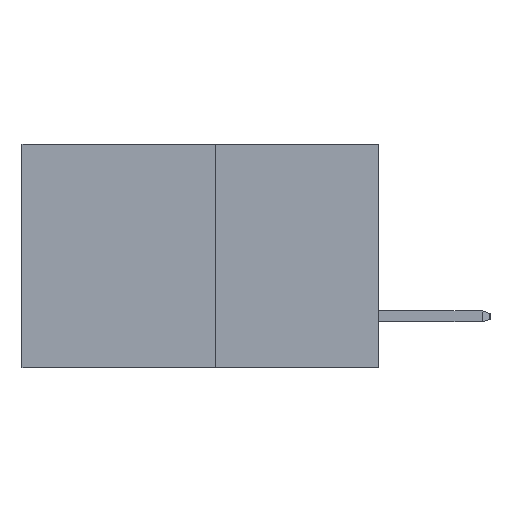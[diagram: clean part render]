
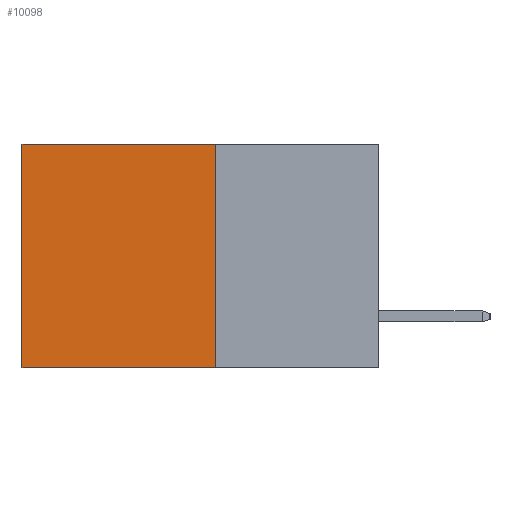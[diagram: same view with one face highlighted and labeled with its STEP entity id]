
A CAD part, left-side view. The second image highlights one B-rep face of the part: STEP entity #10098.
In plain terms, the highlighted planar face has unit normal (-1, 0, 0).
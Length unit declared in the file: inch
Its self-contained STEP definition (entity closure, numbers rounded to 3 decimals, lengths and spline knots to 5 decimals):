
#211 = CARTESIAN_POINT ( 'NONE',  ( 0.277, 0.27, -0.37 ) ) ;
#232 = VERTEX_POINT ( 'NONE', #278 ) ;
#278 = CARTESIAN_POINT ( 'NONE',  ( 0.277, 0.27, 0. ) ) ;
#397 = VECTOR ( 'NONE', #10402, 39.37008 ) ;
#844 = VERTEX_POINT ( 'NONE', #7698 ) ;
#1536 = VERTEX_POINT ( 'NONE', #6334 ) ;
#2068 = CARTESIAN_POINT ( 'NONE',  ( 0.277, 0.27, -0.37 ) ) ;
#2429 = EDGE_CURVE ( 'NONE', #232, #1536, #5053, .T. ) ;
#3121 = CARTESIAN_POINT ( 'NONE',  ( 0.277, 0.59, -0.37 ) ) ;
#3392 = ORIENTED_EDGE ( 'NONE', *, *, #4821, .T. ) ;
#3768 = VECTOR ( 'NONE', #6677, 39.37008 ) ;
#4328 = DIRECTION ( 'NONE',  ( 1., 0., 0. ) ) ;
#4422 = FACE_OUTER_BOUND ( 'NONE', #8122, .T. ) ;
#4745 = EDGE_CURVE ( 'NONE', #232, #7334, #8312, .T. ) ;
#4821 = EDGE_CURVE ( 'NONE', #1536, #844, #9881, .T. ) ;
#5053 = LINE ( 'NONE', #8306, #7510 ) ;
#5304 = ORIENTED_EDGE ( 'NONE', *, *, #4745, .F. ) ;
#5486 = DIRECTION ( 'NONE',  ( 0., 1., 0. ) ) ;
#6055 = AXIS2_PLACEMENT_3D ( 'NONE', #9775, #4328, #10689 ) ;
#6334 = CARTESIAN_POINT ( 'NONE',  ( 0.277, 0.59, 0. ) ) ;
#6677 = DIRECTION ( 'NONE',  ( 0., 0., -1. ) ) ;
#7334 = VERTEX_POINT ( 'NONE', #2068 ) ;
#7510 = VECTOR ( 'NONE', #11266, 39.37008 ) ;
#7698 = CARTESIAN_POINT ( 'NONE',  ( 0.277, 0.59, -0.37 ) ) ;
#7940 = PLANE ( 'NONE',  #6055 ) ;
#8122 = EDGE_LOOP ( 'NONE', ( #3392, #11118, #5304, #11202 ) ) ;
#8306 = CARTESIAN_POINT ( 'NONE',  ( 0.277, 0.27, 0. ) ) ;
#8312 = LINE ( 'NONE', #211, #3768 ) ;
#8406 = EDGE_CURVE ( 'NONE', #7334, #844, #9588, .T. ) ;
#9105 = CARTESIAN_POINT ( 'NONE',  ( 0.277, 0.27, -0.37 ) ) ;
#9304 = VECTOR ( 'NONE', #5486, 39.37008 ) ;
#9588 = LINE ( 'NONE', #9105, #9304 ) ;
#9775 = CARTESIAN_POINT ( 'NONE',  ( 0.277, 0.27, -0.37 ) ) ;
#9881 = LINE ( 'NONE', #3121, #397 ) ;
#10098 = ADVANCED_FACE ( 'NONE', ( #4422 ), #7940, .F. ) ;
#10402 = DIRECTION ( 'NONE',  ( 0., 0., -1. ) ) ;
#10689 = DIRECTION ( 'NONE',  ( 0., 0., -1. ) ) ;
#11118 = ORIENTED_EDGE ( 'NONE', *, *, #8406, .F. ) ;
#11202 = ORIENTED_EDGE ( 'NONE', *, *, #2429, .T. ) ;
#11266 = DIRECTION ( 'NONE',  ( 0., 1., 0. ) ) ;
